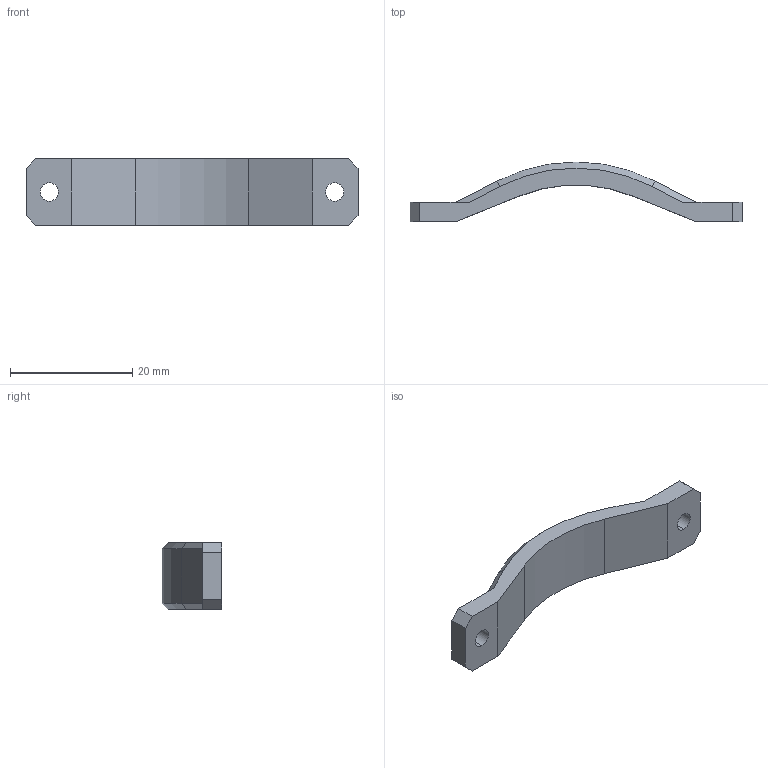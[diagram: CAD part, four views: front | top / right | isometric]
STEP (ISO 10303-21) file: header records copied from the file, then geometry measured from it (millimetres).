
FILE_DESCRIPTION (( 'STEP AP214' ), '1' );
FILE_NAME ('Thunderbolt_Trigger_Guard.STEP', '2021-09-12T03:48:03', ( '' ), ( '' ), 'SwSTEP 2.0', 'SolidWorks 2020', '' );
FILE_SCHEMA (( 'AUTOMOTIVE_DESIGN' ));
Length unit declared in the file: millimetre
Products named in the file (1): Thunderbolt_Trigger_Guard
Bounding box: 54.31 x 9.79 x 10.92 mm (x, y, z)
Volume: 2037 mm3; surface area: 1662.6 mm2
Topology: 1 solids, 1 shells, 28 faces, 74 edges, 48 vertices
Faces by surface type: plane 20, cylinder 6, cone 2
Entity records: 902 total; most frequent: CARTESIAN_POINT 151, ORIENTED_EDGE 148, DIRECTION 146, EDGE_CURVE 74, VECTOR 60, LINE 60, VERTEX_POINT 48, AXIS2_PLACEMENT_3D 43
